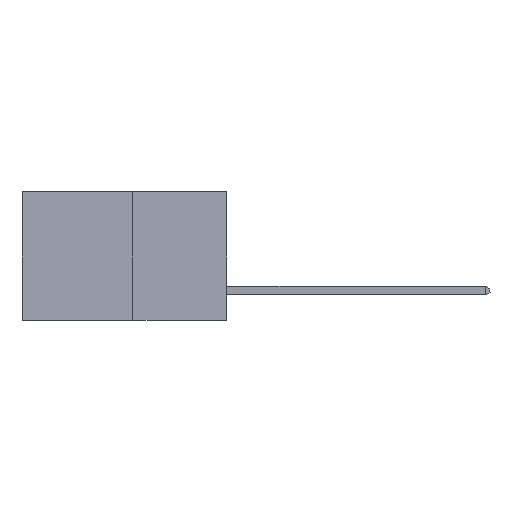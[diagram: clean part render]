
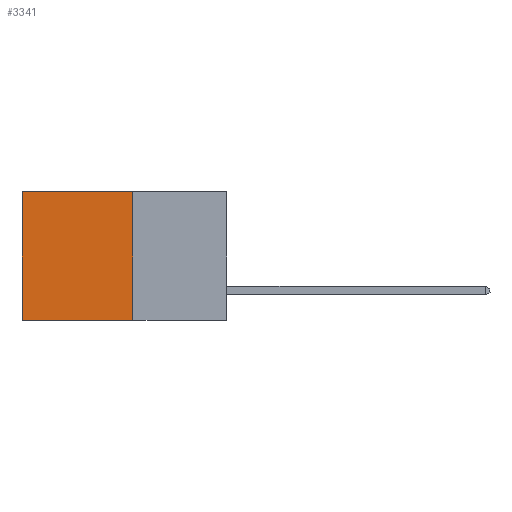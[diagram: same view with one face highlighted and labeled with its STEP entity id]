
A CAD part, left-side view. The second image highlights one B-rep face of the part: STEP entity #3341.
In plain terms, the highlighted planar face has unit normal (-1, 0, 0).
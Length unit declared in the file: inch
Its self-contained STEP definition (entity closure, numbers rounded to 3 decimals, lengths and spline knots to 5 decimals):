
#35 = CARTESIAN_POINT ( 'NONE',  ( 0.277, 0.27, -0.37 ) ) ;
#137 = CARTESIAN_POINT ( 'NONE',  ( 0.277, 0.27, -0.37 ) ) ;
#1028 = ORIENTED_EDGE ( 'NONE', *, *, #14522, .T. ) ;
#1089 = VECTOR ( 'NONE', #6452, 39.37008 ) ;
#1378 = CARTESIAN_POINT ( 'NONE',  ( 0.277, 0.59, 0. ) ) ;
#2727 = CARTESIAN_POINT ( 'NONE',  ( 0.277, 0.27, 0. ) ) ;
#3341 = ADVANCED_FACE ( 'NONE', ( #16557 ), #16091, .F. ) ;
#3363 = DIRECTION ( 'NONE',  ( 0., 0., -1. ) ) ;
#4114 = EDGE_CURVE ( 'NONE', #7290, #16217, #18274, .T. ) ;
#5006 = CARTESIAN_POINT ( 'NONE',  ( 0.277, 0.27, 0. ) ) ;
#5295 = VECTOR ( 'NONE', #8671, 39.37008 ) ;
#6452 = DIRECTION ( 'NONE',  ( 0., 0., -1. ) ) ;
#7244 = ORIENTED_EDGE ( 'NONE', *, *, #7799, .F. ) ;
#7290 = VERTEX_POINT ( 'NONE', #2727 ) ;
#7339 = AXIS2_PLACEMENT_3D ( 'NONE', #7580, #11856, #3363 ) ;
#7580 = CARTESIAN_POINT ( 'NONE',  ( 0.277, 0.27, -0.37 ) ) ;
#7677 = ORIENTED_EDGE ( 'NONE', *, *, #17082, .F. ) ;
#7799 = EDGE_CURVE ( 'NONE', #7290, #13709, #12835, .T. ) ;
#7864 = DIRECTION ( 'NONE',  ( 0., 1., 0. ) ) ;
#7872 = EDGE_LOOP ( 'NONE', ( #1028, #7677, #7244, #12640 ) ) ;
#8162 = LINE ( 'NONE', #14945, #1089 ) ;
#8671 = DIRECTION ( 'NONE',  ( 0., 0., -1. ) ) ;
#9704 = VERTEX_POINT ( 'NONE', #9846 ) ;
#9846 = CARTESIAN_POINT ( 'NONE',  ( 0.277, 0.59, -0.37 ) ) ;
#11856 = DIRECTION ( 'NONE',  ( 1., 0., 0. ) ) ;
#12528 = VECTOR ( 'NONE', #16901, 39.37008 ) ;
#12640 = ORIENTED_EDGE ( 'NONE', *, *, #4114, .T. ) ;
#12662 = CARTESIAN_POINT ( 'NONE',  ( 0.277, 0.27, -0.37 ) ) ;
#12835 = LINE ( 'NONE', #137, #5295 ) ;
#12996 = LINE ( 'NONE', #12662, #12528 ) ;
#13709 = VERTEX_POINT ( 'NONE', #35 ) ;
#14512 = VECTOR ( 'NONE', #7864, 39.37008 ) ;
#14522 = EDGE_CURVE ( 'NONE', #16217, #9704, #8162, .T. ) ;
#14945 = CARTESIAN_POINT ( 'NONE',  ( 0.277, 0.59, -0.37 ) ) ;
#16091 = PLANE ( 'NONE',  #7339 ) ;
#16217 = VERTEX_POINT ( 'NONE', #1378 ) ;
#16557 = FACE_OUTER_BOUND ( 'NONE', #7872, .T. ) ;
#16901 = DIRECTION ( 'NONE',  ( 0., 1., 0. ) ) ;
#17082 = EDGE_CURVE ( 'NONE', #13709, #9704, #12996, .T. ) ;
#18274 = LINE ( 'NONE', #5006, #14512 ) ;
